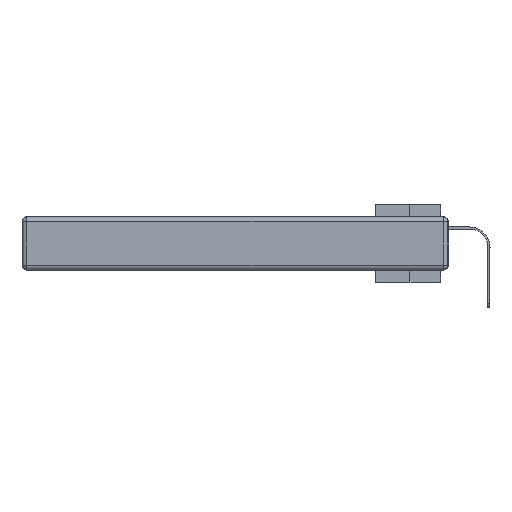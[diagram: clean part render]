
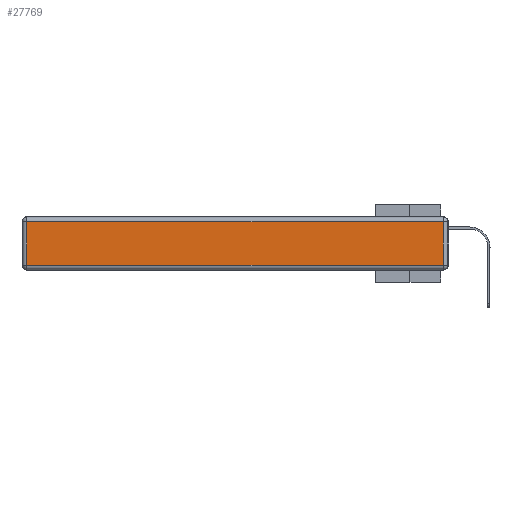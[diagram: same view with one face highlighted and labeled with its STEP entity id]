
A CAD part, left-side view. The second image highlights one B-rep face of the part: STEP entity #27769.
In plain terms, the highlighted planar face has unit normal (-1, 0, 0).
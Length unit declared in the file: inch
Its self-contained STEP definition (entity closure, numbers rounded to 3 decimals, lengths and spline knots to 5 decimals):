
#285 = DIRECTION ( 'NONE',  ( 0., 0., -1. ) ) ;
#739 = LINE ( 'NONE', #23465, #4108 ) ;
#1491 = DIRECTION ( 'NONE',  ( 0., -1., 0. ) ) ;
#1691 = DIRECTION ( 'NONE',  ( 0., 0., 1. ) ) ;
#3475 = AXIS2_PLACEMENT_3D ( 'NONE', #19538, #22042, #1691 ) ;
#3917 = EDGE_CURVE ( 'NONE', #21677, #19515, #8348, .T. ) ;
#4012 = CARTESIAN_POINT ( 'NONE',  ( 0., 0.03, -0.03 ) ) ;
#4108 = VECTOR ( 'NONE', #12211, 39.37008 ) ;
#5621 = ORIENTED_EDGE ( 'NONE', *, *, #3917, .T. ) ;
#6185 = FACE_OUTER_BOUND ( 'NONE', #6711, .T. ) ;
#6640 = EDGE_CURVE ( 'NONE', #19515, #12592, #739, .T. ) ;
#6711 = EDGE_LOOP ( 'NONE', ( #5621, #18893, #17425, #12357 ) ) ;
#8348 = LINE ( 'NONE', #12946, #28628 ) ;
#8925 = DIRECTION ( 'NONE',  ( 0., 1., 0. ) ) ;
#9536 = CARTESIAN_POINT ( 'NONE',  ( 0., 2.72, -0.343 ) ) ;
#10513 = PLANE ( 'NONE',  #3475 ) ;
#10724 = CARTESIAN_POINT ( 'NONE',  ( 0., 0.03, -0.313 ) ) ;
#12211 = DIRECTION ( 'NONE',  ( 0., 0., 1. ) ) ;
#12357 = ORIENTED_EDGE ( 'NONE', *, *, #13915, .T. ) ;
#12592 = VERTEX_POINT ( 'NONE', #4012 ) ;
#12946 = CARTESIAN_POINT ( 'NONE',  ( 0., 0., -0.313 ) ) ;
#13915 = EDGE_CURVE ( 'NONE', #17359, #21677, #27605, .T. ) ;
#17359 = VERTEX_POINT ( 'NONE', #26313 ) ;
#17406 = EDGE_CURVE ( 'NONE', #12592, #17359, #20617, .T. ) ;
#17425 = ORIENTED_EDGE ( 'NONE', *, *, #17406, .T. ) ;
#18539 = CARTESIAN_POINT ( 'NONE',  ( 0., 2.75, -0.03 ) ) ;
#18893 = ORIENTED_EDGE ( 'NONE', *, *, #6640, .T. ) ;
#19515 = VERTEX_POINT ( 'NONE', #10724 ) ;
#19538 = CARTESIAN_POINT ( 'NONE',  ( 0., 0., -0.343 ) ) ;
#20617 = LINE ( 'NONE', #18539, #21202 ) ;
#21202 = VECTOR ( 'NONE', #8925, 39.37008 ) ;
#21677 = VERTEX_POINT ( 'NONE', #29129 ) ;
#22042 = DIRECTION ( 'NONE',  ( -1., 0., 0. ) ) ;
#23465 = CARTESIAN_POINT ( 'NONE',  ( 0., 0.03, -0.343 ) ) ;
#26313 = CARTESIAN_POINT ( 'NONE',  ( 0., 2.72, -0.03 ) ) ;
#27605 = LINE ( 'NONE', #9536, #27736 ) ;
#27736 = VECTOR ( 'NONE', #285, 39.37008 ) ;
#27769 = ADVANCED_FACE ( 'NONE', ( #6185 ), #10513, .T. ) ;
#28628 = VECTOR ( 'NONE', #1491, 39.37008 ) ;
#29129 = CARTESIAN_POINT ( 'NONE',  ( 0., 2.72, -0.313 ) ) ;
